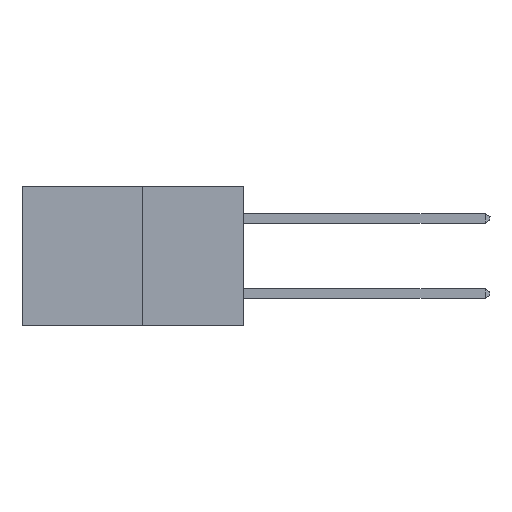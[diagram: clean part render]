
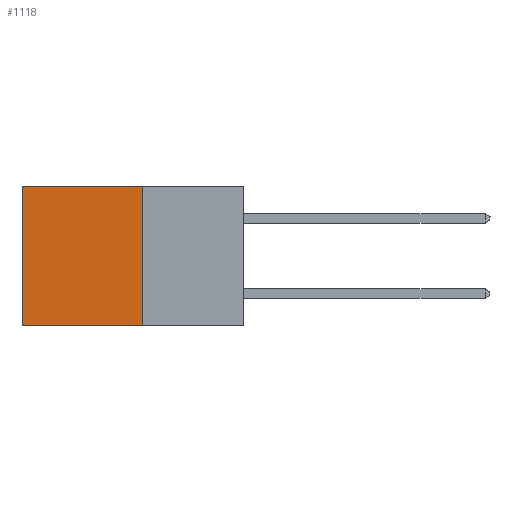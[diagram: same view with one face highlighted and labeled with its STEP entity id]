
A CAD part, left-side view. The second image highlights one B-rep face of the part: STEP entity #1118.
In plain terms, the highlighted planar face has unit normal (-1, 0, 0).
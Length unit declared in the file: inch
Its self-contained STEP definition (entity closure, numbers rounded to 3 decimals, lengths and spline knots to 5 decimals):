
#1118 = ADVANCED_FACE ( 'NONE', ( #11614 ), #6806, .F. ) ;
#1369 = CARTESIAN_POINT ( 'NONE',  ( 0.277, 0.59, 0. ) ) ;
#1499 = LINE ( 'NONE', #8613, #7616 ) ;
#2094 = CARTESIAN_POINT ( 'NONE',  ( 0.277, 0.27, -0.37 ) ) ;
#2367 = EDGE_CURVE ( 'NONE', #12456, #8845, #12649, .T. ) ;
#3027 = VERTEX_POINT ( 'NONE', #9608 ) ;
#3429 = EDGE_LOOP ( 'NONE', ( #12868, #10131, #4240, #6763 ) ) ;
#4240 = ORIENTED_EDGE ( 'NONE', *, *, #8677, .F. ) ;
#5616 = CARTESIAN_POINT ( 'NONE',  ( 0.277, 0.27, 0. ) ) ;
#6343 = VECTOR ( 'NONE', #6743, 39.37008 ) ;
#6712 = CARTESIAN_POINT ( 'NONE',  ( 0.277, 0.59, -0.37 ) ) ;
#6743 = DIRECTION ( 'NONE',  ( 0., 0., -1. ) ) ;
#6763 = ORIENTED_EDGE ( 'NONE', *, *, #11506, .T. ) ;
#6806 = PLANE ( 'NONE',  #7226 ) ;
#7226 = AXIS2_PLACEMENT_3D ( 'NONE', #14005, #12664, #12622 ) ;
#7481 = EDGE_CURVE ( 'NONE', #10975, #8845, #1499, .T. ) ;
#7567 = DIRECTION ( 'NONE',  ( 0., 1., 0. ) ) ;
#7616 = VECTOR ( 'NONE', #7567, 39.37008 ) ;
#8251 = VECTOR ( 'NONE', #13890, 39.37008 ) ;
#8613 = CARTESIAN_POINT ( 'NONE',  ( 0.277, 0.27, -0.37 ) ) ;
#8677 = EDGE_CURVE ( 'NONE', #3027, #10975, #13150, .T. ) ;
#8845 = VERTEX_POINT ( 'NONE', #10718 ) ;
#9608 = CARTESIAN_POINT ( 'NONE',  ( 0.277, 0.27, 0. ) ) ;
#10131 = ORIENTED_EDGE ( 'NONE', *, *, #7481, .F. ) ;
#10248 = DIRECTION ( 'NONE',  ( 0., 0., -1. ) ) ;
#10718 = CARTESIAN_POINT ( 'NONE',  ( 0.277, 0.59, -0.37 ) ) ;
#10975 = VERTEX_POINT ( 'NONE', #12938 ) ;
#11506 = EDGE_CURVE ( 'NONE', #3027, #12456, #14191, .T. ) ;
#11614 = FACE_OUTER_BOUND ( 'NONE', #3429, .T. ) ;
#12456 = VERTEX_POINT ( 'NONE', #1369 ) ;
#12622 = DIRECTION ( 'NONE',  ( 0., 0., -1. ) ) ;
#12649 = LINE ( 'NONE', #6712, #6343 ) ;
#12664 = DIRECTION ( 'NONE',  ( 1., 0., 0. ) ) ;
#12868 = ORIENTED_EDGE ( 'NONE', *, *, #2367, .T. ) ;
#12938 = CARTESIAN_POINT ( 'NONE',  ( 0.277, 0.27, -0.37 ) ) ;
#13150 = LINE ( 'NONE', #2094, #14792 ) ;
#13890 = DIRECTION ( 'NONE',  ( 0., 1., 0. ) ) ;
#14005 = CARTESIAN_POINT ( 'NONE',  ( 0.277, 0.27, -0.37 ) ) ;
#14191 = LINE ( 'NONE', #5616, #8251 ) ;
#14792 = VECTOR ( 'NONE', #10248, 39.37008 ) ;
